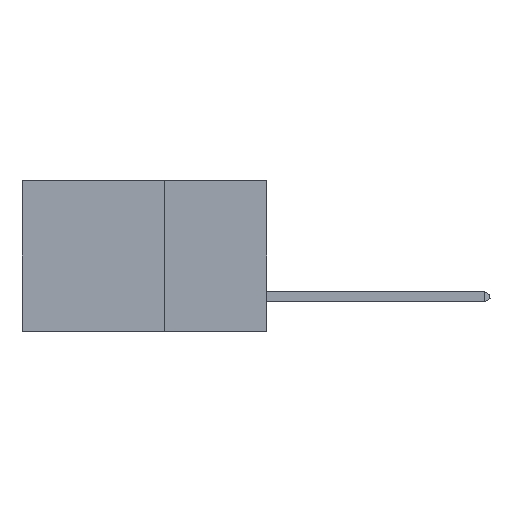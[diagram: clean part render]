
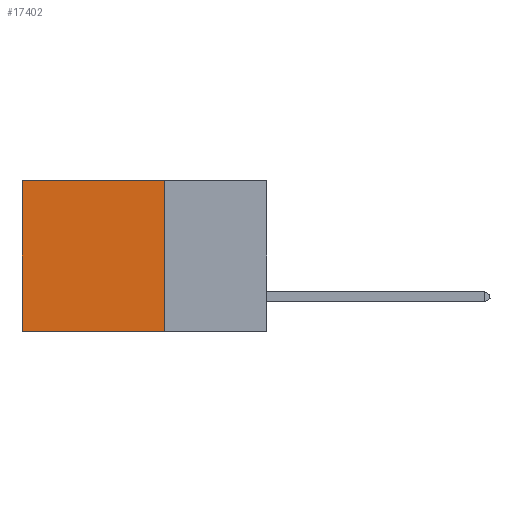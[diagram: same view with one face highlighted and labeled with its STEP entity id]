
A CAD part, left-side view. The second image highlights one B-rep face of the part: STEP entity #17402.
In plain terms, the highlighted planar face has unit normal (-1, 0, 0).
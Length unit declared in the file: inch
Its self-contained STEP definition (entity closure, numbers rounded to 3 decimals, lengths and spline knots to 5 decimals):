
#401 = VERTEX_POINT ( 'NONE', #18583 ) ;
#4167 = ORIENTED_EDGE ( 'NONE', *, *, #9341, .F. ) ;
#4468 = EDGE_CURVE ( 'NONE', #8805, #401, #23720, .T. ) ;
#4774 = LINE ( 'NONE', #19800, #24567 ) ;
#5718 = VERTEX_POINT ( 'NONE', #5819 ) ;
#5819 = CARTESIAN_POINT ( 'NONE',  ( 0.2875, 0.6, -0.37 ) ) ;
#6571 = VECTOR ( 'NONE', #8796, 39.37008 ) ;
#6631 = EDGE_CURVE ( 'NONE', #401, #5718, #19146, .T. ) ;
#8535 = ORIENTED_EDGE ( 'NONE', *, *, #6631, .T. ) ;
#8702 = EDGE_CURVE ( 'NONE', #8805, #17522, #9711, .T. ) ;
#8796 = DIRECTION ( 'NONE',  ( 0., 0., -1. ) ) ;
#8805 = VERTEX_POINT ( 'NONE', #15232 ) ;
#9341 = EDGE_CURVE ( 'NONE', #17522, #5718, #4774, .T. ) ;
#9711 = LINE ( 'NONE', #14210, #18712 ) ;
#10393 = ORIENTED_EDGE ( 'NONE', *, *, #8702, .F. ) ;
#12744 = DIRECTION ( 'NONE',  ( 0., 1., 0. ) ) ;
#14025 = DIRECTION ( 'NONE',  ( 0., 1., 0. ) ) ;
#14210 = CARTESIAN_POINT ( 'NONE',  ( 0.2875, 0.25, 0. ) ) ;
#14382 = AXIS2_PLACEMENT_3D ( 'NONE', #24500, #16809, #24406 ) ;
#14805 = ORIENTED_EDGE ( 'NONE', *, *, #4468, .T. ) ;
#15232 = CARTESIAN_POINT ( 'NONE',  ( 0.2875, 0.25, 0. ) ) ;
#16719 = PLANE ( 'NONE',  #14382 ) ;
#16809 = DIRECTION ( 'NONE',  ( 1., 0., 0. ) ) ;
#17402 = ADVANCED_FACE ( 'NONE', ( #21261 ), #16719, .F. ) ;
#17522 = VERTEX_POINT ( 'NONE', #23578 ) ;
#18435 = CARTESIAN_POINT ( 'NONE',  ( 0.2875, 0.25, 0. ) ) ;
#18583 = CARTESIAN_POINT ( 'NONE',  ( 0.2875, 0.6, 0. ) ) ;
#18712 = VECTOR ( 'NONE', #19818, 39.37008 ) ;
#19146 = LINE ( 'NONE', #22611, #6571 ) ;
#19800 = CARTESIAN_POINT ( 'NONE',  ( 0.2875, 0.25, -0.37 ) ) ;
#19818 = DIRECTION ( 'NONE',  ( 0., 0., -1. ) ) ;
#21261 = FACE_OUTER_BOUND ( 'NONE', #24556, .T. ) ;
#22527 = VECTOR ( 'NONE', #12744, 39.37008 ) ;
#22611 = CARTESIAN_POINT ( 'NONE',  ( 0.2875, 0.6, 0. ) ) ;
#23578 = CARTESIAN_POINT ( 'NONE',  ( 0.2875, 0.25, -0.37 ) ) ;
#23720 = LINE ( 'NONE', #18435, #22527 ) ;
#24406 = DIRECTION ( 'NONE',  ( 0., 0., -1. ) ) ;
#24500 = CARTESIAN_POINT ( 'NONE',  ( 0.2875, 0.25, 0. ) ) ;
#24556 = EDGE_LOOP ( 'NONE', ( #8535, #4167, #10393, #14805 ) ) ;
#24567 = VECTOR ( 'NONE', #14025, 39.37008 ) ;
